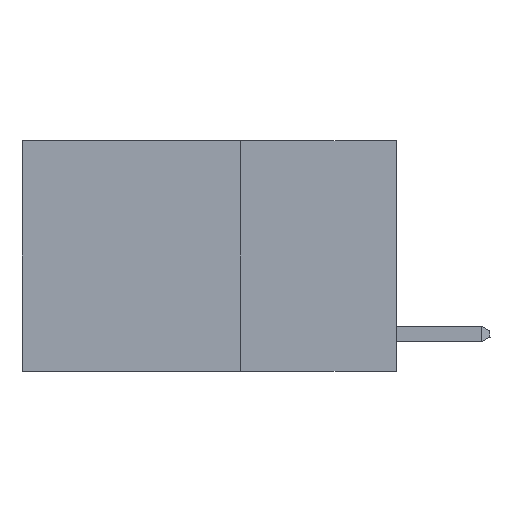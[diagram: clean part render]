
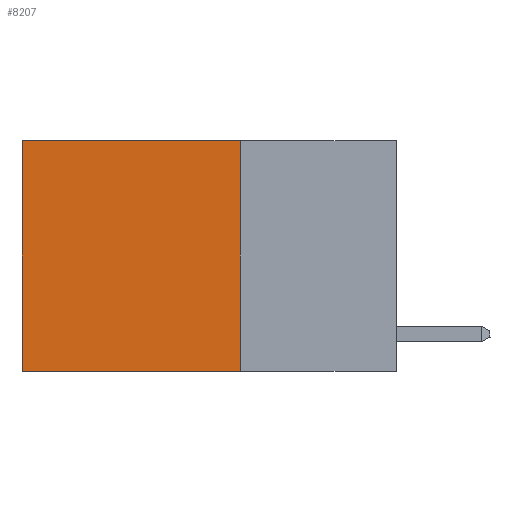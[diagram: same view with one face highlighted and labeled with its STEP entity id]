
A CAD part, left-side view. The second image highlights one B-rep face of the part: STEP entity #8207.
In plain terms, the highlighted planar face has unit normal (-1, 0, 0).
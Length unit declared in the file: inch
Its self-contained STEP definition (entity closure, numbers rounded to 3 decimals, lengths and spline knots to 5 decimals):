
#70 = DIRECTION ( 'NONE',  ( 0., 1., 0. ) ) ;
#255 = EDGE_CURVE ( 'NONE', #11547, #10182, #11137, .T. ) ;
#302 = PLANE ( 'NONE',  #3483 ) ;
#600 = CARTESIAN_POINT ( 'NONE',  ( 0.2625, 0.25, -0.37 ) ) ;
#1302 = VECTOR ( 'NONE', #7657, 39.37008 ) ;
#1838 = ORIENTED_EDGE ( 'NONE', *, *, #4325, .T. ) ;
#2604 = CARTESIAN_POINT ( 'NONE',  ( 0.2625, 0.6, 0. ) ) ;
#2960 = CARTESIAN_POINT ( 'NONE',  ( 0.2625, 0.25, 0. ) ) ;
#3046 = ORIENTED_EDGE ( 'NONE', *, *, #7521, .F. ) ;
#3175 = DIRECTION ( 'NONE',  ( 0., 0., -1. ) ) ;
#3483 = AXIS2_PLACEMENT_3D ( 'NONE', #4121, #7954, #3175 ) ;
#3515 = DIRECTION ( 'NONE',  ( 0., 0., -1. ) ) ;
#4008 = LINE ( 'NONE', #4761, #1302 ) ;
#4035 = VECTOR ( 'NONE', #7509, 39.37008 ) ;
#4121 = CARTESIAN_POINT ( 'NONE',  ( 0.2625, 0.25, 0. ) ) ;
#4273 = CARTESIAN_POINT ( 'NONE',  ( 0.2625, 0.25, 0. ) ) ;
#4325 = EDGE_CURVE ( 'NONE', #4502, #11547, #9797, .T. ) ;
#4502 = VERTEX_POINT ( 'NONE', #12005 ) ;
#4761 = CARTESIAN_POINT ( 'NONE',  ( 0.2625, 0.25, -0.37 ) ) ;
#7509 = DIRECTION ( 'NONE',  ( 0., 0., -1. ) ) ;
#7521 = EDGE_CURVE ( 'NONE', #9097, #10182, #4008, .T. ) ;
#7657 = DIRECTION ( 'NONE',  ( 0., 1., 0. ) ) ;
#7954 = DIRECTION ( 'NONE',  ( 1., 0., 0. ) ) ;
#8207 = ADVANCED_FACE ( 'NONE', ( #8895 ), #302, .F. ) ;
#8895 = FACE_OUTER_BOUND ( 'NONE', #10578, .T. ) ;
#9053 = LINE ( 'NONE', #4273, #9501 ) ;
#9097 = VERTEX_POINT ( 'NONE', #600 ) ;
#9132 = EDGE_CURVE ( 'NONE', #4502, #9097, #9053, .T. ) ;
#9501 = VECTOR ( 'NONE', #3515, 39.37008 ) ;
#9797 = LINE ( 'NONE', #2960, #10356 ) ;
#9820 = CARTESIAN_POINT ( 'NONE',  ( 0.2625, 0.6, -0.37 ) ) ;
#10009 = CARTESIAN_POINT ( 'NONE',  ( 0.2625, 0.6, 0. ) ) ;
#10182 = VERTEX_POINT ( 'NONE', #9820 ) ;
#10356 = VECTOR ( 'NONE', #70, 39.37008 ) ;
#10578 = EDGE_LOOP ( 'NONE', ( #11317, #3046, #10975, #1838 ) ) ;
#10975 = ORIENTED_EDGE ( 'NONE', *, *, #9132, .F. ) ;
#11137 = LINE ( 'NONE', #2604, #4035 ) ;
#11317 = ORIENTED_EDGE ( 'NONE', *, *, #255, .T. ) ;
#11547 = VERTEX_POINT ( 'NONE', #10009 ) ;
#12005 = CARTESIAN_POINT ( 'NONE',  ( 0.2625, 0.25, 0. ) ) ;
